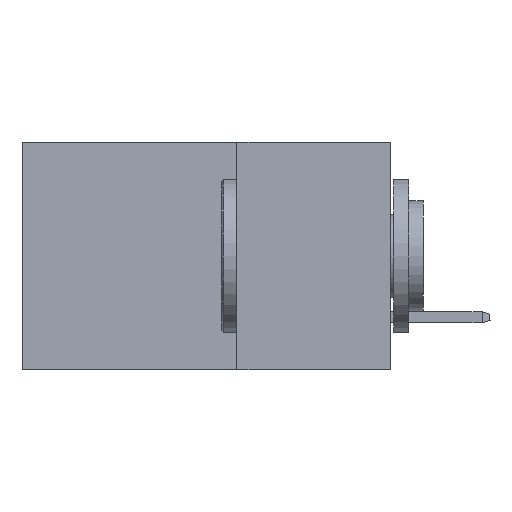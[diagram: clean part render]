
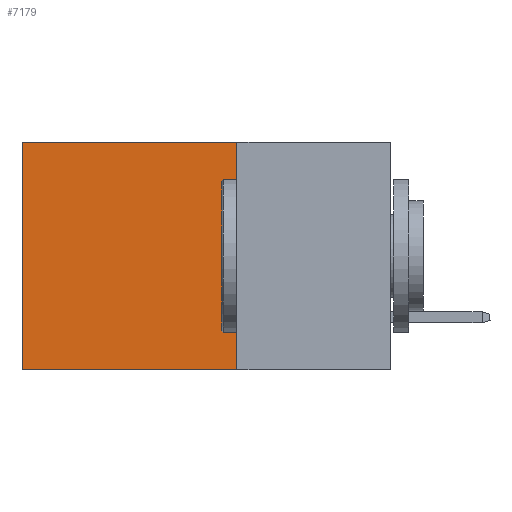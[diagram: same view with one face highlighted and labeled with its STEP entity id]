
A CAD part, left-side view. The second image highlights one B-rep face of the part: STEP entity #7179.
In plain terms, the highlighted planar face has unit normal (-1, 0, 0).
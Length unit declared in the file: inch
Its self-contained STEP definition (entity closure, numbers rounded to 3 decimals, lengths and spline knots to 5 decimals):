
#135 = ORIENTED_EDGE ( 'NONE', *, *, #912, .T. ) ;
#912 = EDGE_CURVE ( 'NONE', #32162, #30708, #7295, .T. ) ;
#1457 = EDGE_LOOP ( 'NONE', ( #19919, #24269, #3369, #135 ) ) ;
#1707 = CARTESIAN_POINT ( 'NONE',  ( 0.2875, 0.6, 0. ) ) ;
#2755 = CARTESIAN_POINT ( 'NONE',  ( 0.2875, 0.25, 0. ) ) ;
#3009 = CARTESIAN_POINT ( 'NONE',  ( 0.2875, 0.25, -0.37 ) ) ;
#3369 = ORIENTED_EDGE ( 'NONE', *, *, #6871, .F. ) ;
#3694 = VECTOR ( 'NONE', #9218, 39.37008 ) ;
#4366 = CARTESIAN_POINT ( 'NONE',  ( 0.2875, 0.25, 0. ) ) ;
#5348 = DIRECTION ( 'NONE',  ( 0., 0., -1. ) ) ;
#6620 = EDGE_CURVE ( 'NONE', #22617, #9429, #24771, .T. ) ;
#6871 = EDGE_CURVE ( 'NONE', #32162, #22617, #30438, .T. ) ;
#7179 = ADVANCED_FACE ( 'NONE', ( #19912 ), #31152, .F. ) ;
#7295 = LINE ( 'NONE', #17054, #13392 ) ;
#9218 = DIRECTION ( 'NONE',  ( 0., 0., -1. ) ) ;
#9429 = VERTEX_POINT ( 'NONE', #25124 ) ;
#10850 = CARTESIAN_POINT ( 'NONE',  ( 0.2875, 0.6, 0. ) ) ;
#11829 = DIRECTION ( 'NONE',  ( 0., 1., 0. ) ) ;
#13392 = VECTOR ( 'NONE', #11829, 39.37008 ) ;
#16167 = DIRECTION ( 'NONE',  ( 0., 0., -1. ) ) ;
#17054 = CARTESIAN_POINT ( 'NONE',  ( 0.2875, 0.25, 0. ) ) ;
#17565 = VECTOR ( 'NONE', #16167, 39.37008 ) ;
#17919 = VECTOR ( 'NONE', #26083, 39.37008 ) ;
#19209 = EDGE_CURVE ( 'NONE', #30708, #9429, #26875, .T. ) ;
#19912 = FACE_OUTER_BOUND ( 'NONE', #1457, .T. ) ;
#19919 = ORIENTED_EDGE ( 'NONE', *, *, #19209, .T. ) ;
#20296 = AXIS2_PLACEMENT_3D ( 'NONE', #2755, #20840, #5348 ) ;
#20840 = DIRECTION ( 'NONE',  ( 1., 0., 0. ) ) ;
#22334 = CARTESIAN_POINT ( 'NONE',  ( 0.2875, 0.25, -0.37 ) ) ;
#22617 = VERTEX_POINT ( 'NONE', #22334 ) ;
#24269 = ORIENTED_EDGE ( 'NONE', *, *, #6620, .F. ) ;
#24771 = LINE ( 'NONE', #3009, #17919 ) ;
#25124 = CARTESIAN_POINT ( 'NONE',  ( 0.2875, 0.6, -0.37 ) ) ;
#26083 = DIRECTION ( 'NONE',  ( 0., 1., 0. ) ) ;
#26875 = LINE ( 'NONE', #10850, #17565 ) ;
#27322 = CARTESIAN_POINT ( 'NONE',  ( 0.2875, 0.25, 0. ) ) ;
#30438 = LINE ( 'NONE', #27322, #3694 ) ;
#30708 = VERTEX_POINT ( 'NONE', #1707 ) ;
#31152 = PLANE ( 'NONE',  #20296 ) ;
#32162 = VERTEX_POINT ( 'NONE', #4366 ) ;
